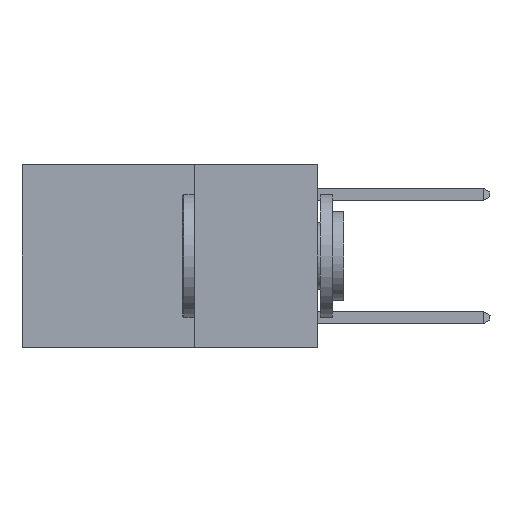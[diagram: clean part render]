
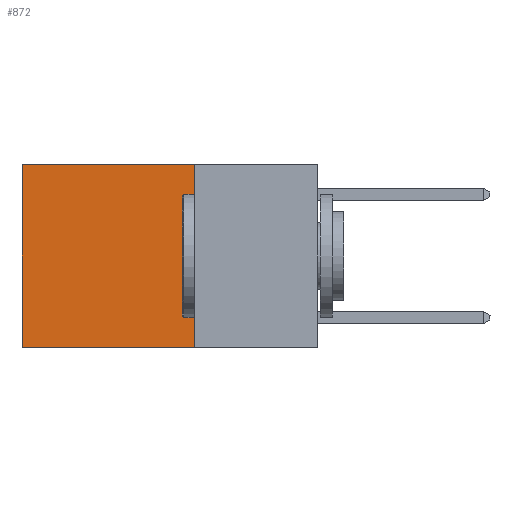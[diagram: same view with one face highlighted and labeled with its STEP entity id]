
A CAD part, left-side view. The second image highlights one B-rep face of the part: STEP entity #872.
In plain terms, the highlighted planar face has unit normal (-1, 0, 0).
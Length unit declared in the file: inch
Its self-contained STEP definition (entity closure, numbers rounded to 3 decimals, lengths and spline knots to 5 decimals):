
#342 = EDGE_CURVE ( 'NONE', #2373, #9257, #5040, .T. ) ;
#872 = ADVANCED_FACE ( 'NONE', ( #5291 ), #8501, .F. ) ;
#2138 = VECTOR ( 'NONE', #10759, 39.37008 ) ;
#2230 = VECTOR ( 'NONE', #4887, 39.37008 ) ;
#2373 = VERTEX_POINT ( 'NONE', #5168 ) ;
#2404 = ORIENTED_EDGE ( 'NONE', *, *, #8078, .T. ) ;
#3767 = CARTESIAN_POINT ( 'NONE',  ( 0.2625, 0.6, -0.37 ) ) ;
#4064 = CARTESIAN_POINT ( 'NONE',  ( 0.2625, 0.25, 0. ) ) ;
#4303 = ORIENTED_EDGE ( 'NONE', *, *, #7233, .T. ) ;
#4887 = DIRECTION ( 'NONE',  ( 0., 1., 0. ) ) ;
#4997 = VECTOR ( 'NONE', #8951, 39.37008 ) ;
#5040 = LINE ( 'NONE', #8465, #9089 ) ;
#5168 = CARTESIAN_POINT ( 'NONE',  ( 0.2625, 0.25, 0. ) ) ;
#5182 = VERTEX_POINT ( 'NONE', #6802 ) ;
#5291 = FACE_OUTER_BOUND ( 'NONE', #7436, .T. ) ;
#5566 = CARTESIAN_POINT ( 'NONE',  ( 0.2625, 0.25, -0.37 ) ) ;
#5592 = EDGE_CURVE ( 'NONE', #9257, #10084, #10612, .T. ) ;
#6025 = AXIS2_PLACEMENT_3D ( 'NONE', #8610, #8419, #8407 ) ;
#6450 = DIRECTION ( 'NONE',  ( 0., 0., -1. ) ) ;
#6477 = ORIENTED_EDGE ( 'NONE', *, *, #342, .F. ) ;
#6743 = LINE ( 'NONE', #9951, #2138 ) ;
#6802 = CARTESIAN_POINT ( 'NONE',  ( 0.2625, 0.6, 0. ) ) ;
#7233 = EDGE_CURVE ( 'NONE', #2373, #5182, #9299, .T. ) ;
#7436 = EDGE_LOOP ( 'NONE', ( #2404, #10771, #6477, #4303 ) ) ;
#8078 = EDGE_CURVE ( 'NONE', #5182, #10084, #6743, .T. ) ;
#8407 = DIRECTION ( 'NONE',  ( 0., 0., -1. ) ) ;
#8419 = DIRECTION ( 'NONE',  ( 1., 0., 0. ) ) ;
#8465 = CARTESIAN_POINT ( 'NONE',  ( 0.2625, 0.25, 0. ) ) ;
#8501 = PLANE ( 'NONE',  #6025 ) ;
#8610 = CARTESIAN_POINT ( 'NONE',  ( 0.2625, 0.25, 0. ) ) ;
#8930 = CARTESIAN_POINT ( 'NONE',  ( 0.2625, 0.25, -0.37 ) ) ;
#8951 = DIRECTION ( 'NONE',  ( 0., 1., 0. ) ) ;
#9089 = VECTOR ( 'NONE', #6450, 39.37008 ) ;
#9257 = VERTEX_POINT ( 'NONE', #5566 ) ;
#9299 = LINE ( 'NONE', #4064, #4997 ) ;
#9951 = CARTESIAN_POINT ( 'NONE',  ( 0.2625, 0.6, 0. ) ) ;
#10084 = VERTEX_POINT ( 'NONE', #3767 ) ;
#10612 = LINE ( 'NONE', #8930, #2230 ) ;
#10759 = DIRECTION ( 'NONE',  ( 0., 0., -1. ) ) ;
#10771 = ORIENTED_EDGE ( 'NONE', *, *, #5592, .F. ) ;
